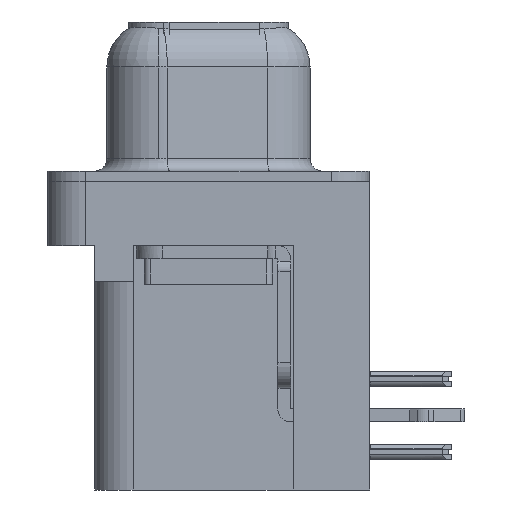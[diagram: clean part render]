
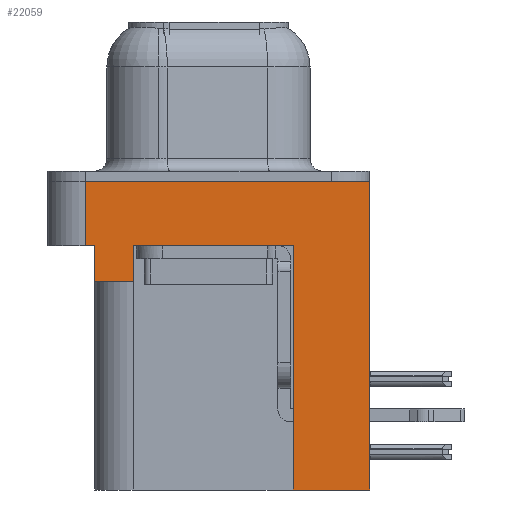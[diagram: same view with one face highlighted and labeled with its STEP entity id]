
A CAD part, left-side view. The second image highlights one B-rep face of the part: STEP entity #22059.
In plain terms, the highlighted planar face has unit normal (-1, 0, 0).
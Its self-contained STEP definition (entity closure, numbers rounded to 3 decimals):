
#230 = DIRECTION ( 'NONE',  ( 0., -1., 0. ) ) ;
#871 = DIRECTION ( 'NONE',  ( -1., 0., 0. ) ) ;
#1240 = DIRECTION ( 'NONE',  ( 0., 0., 1. ) ) ;
#1423 = VECTOR ( 'NONE', #1240, 1000. ) ;
#1454 = LINE ( 'NONE', #35385, #24689 ) ;
#1712 = CARTESIAN_POINT ( 'NONE',  ( -2.91, -3.295, -2.5 ) ) ;
#1952 = VERTEX_POINT ( 'NONE', #25678 ) ;
#1959 = ORIENTED_EDGE ( 'NONE', *, *, #5487, .T. ) ;
#3569 = ORIENTED_EDGE ( 'NONE', *, *, #28888, .F. ) ;
#3679 = LINE ( 'NONE', #10247, #1423 ) ;
#5487 = EDGE_CURVE ( 'NONE', #19455, #36561, #19017, .T. ) ;
#5704 = EDGE_CURVE ( 'NONE', #34224, #36967, #12769, .T. ) ;
#6016 = CARTESIAN_POINT ( 'NONE',  ( -2.91, 2.895, -3.9 ) ) ;
#6312 = EDGE_CURVE ( 'NONE', #34224, #1952, #1454, .T. ) ;
#7328 = EDGE_CURVE ( 'NONE', #1952, #12615, #27888, .T. ) ;
#7333 = EDGE_CURVE ( 'NONE', #30671, #36561, #23378, .T. ) ;
#7464 = DIRECTION ( 'NONE',  ( 0., 0., 1. ) ) ;
#8506 = ORIENTED_EDGE ( 'NONE', *, *, #8767, .F. ) ;
#8767 = EDGE_CURVE ( 'NONE', #19455, #28785, #36981, .T. ) ;
#9227 = ORIENTED_EDGE ( 'NONE', *, *, #5704, .F. ) ;
#9330 = CARTESIAN_POINT ( 'NONE',  ( -2.91, -6.275, 0. ) ) ;
#9486 = VECTOR ( 'NONE', #34793, 1000. ) ;
#9561 = DIRECTION ( 'NONE',  ( 0., 0., 1. ) ) ;
#10042 = VECTOR ( 'NONE', #7464, 1000. ) ;
#10247 = CARTESIAN_POINT ( 'NONE',  ( -2.91, 4.425, -3.9 ) ) ;
#10704 = DIRECTION ( 'NONE',  ( 0., 0., 1. ) ) ;
#10757 = VECTOR ( 'NONE', #230, 1000. ) ;
#11480 = VECTOR ( 'NONE', #15995, 1000. ) ;
#11748 = CARTESIAN_POINT ( 'NONE',  ( -2.91, -6.275, 0. ) ) ;
#12615 = VERTEX_POINT ( 'NONE', #1712 ) ;
#12769 = LINE ( 'NONE', #13774, #26567 ) ;
#12823 = LINE ( 'NONE', #33043, #11480 ) ;
#13774 = CARTESIAN_POINT ( 'NONE',  ( -2.91, 4.425, -3.9 ) ) ;
#14326 = CARTESIAN_POINT ( 'NONE',  ( -2.91, -6.275, -12. ) ) ;
#15126 = ORIENTED_EDGE ( 'NONE', *, *, #29353, .F. ) ;
#15895 = CARTESIAN_POINT ( 'NONE',  ( -2.91, -3.295, -12. ) ) ;
#15995 = DIRECTION ( 'NONE',  ( 0., 0., 1. ) ) ;
#16613 = CARTESIAN_POINT ( 'NONE',  ( -2.91, -6.275, -2.5 ) ) ;
#17686 = VECTOR ( 'NONE', #23473, 1000. ) ;
#18328 = DIRECTION ( 'NONE',  ( 0., 0., 1. ) ) ;
#18672 = ORIENTED_EDGE ( 'NONE', *, *, #7328, .T. ) ;
#18876 = EDGE_LOOP ( 'NONE', ( #28643, #3569, #27681, #15126, #9227, #35859, #18672, #29446, #8506, #1959 ) ) ;
#19017 = LINE ( 'NONE', #16613, #10042 ) ;
#19229 = CARTESIAN_POINT ( 'NONE',  ( -2.91, 4.775, -2.5 ) ) ;
#19455 = VERTEX_POINT ( 'NONE', #14326 ) ;
#20307 = VECTOR ( 'NONE', #10704, 1000. ) ;
#20848 = CARTESIAN_POINT ( 'NONE',  ( -2.91, -6.275, -2.5 ) ) ;
#21636 = FACE_OUTER_BOUND ( 'NONE', #18876, .T. ) ;
#22059 = ADVANCED_FACE ( 'NONE', ( #21636 ), #29882, .T. ) ;
#22552 = CARTESIAN_POINT ( 'NONE',  ( -2.91, -6.275, -2.5 ) ) ;
#23011 = AXIS2_PLACEMENT_3D ( 'NONE', #35419, #871, #9561 ) ;
#23378 = LINE ( 'NONE', #9330, #9486 ) ;
#23473 = DIRECTION ( 'NONE',  ( 0., -1., 0. ) ) ;
#23912 = EDGE_CURVE ( 'NONE', #27477, #36589, #28169, .T. ) ;
#24689 = VECTOR ( 'NONE', #18328, 1000. ) ;
#24942 = DIRECTION ( 'NONE',  ( 0., 1., 0. ) ) ;
#25678 = CARTESIAN_POINT ( 'NONE',  ( -2.91, 2.895, -2.5 ) ) ;
#26457 = CARTESIAN_POINT ( 'NONE',  ( -2.91, -3.295, -12. ) ) ;
#26567 = VECTOR ( 'NONE', #24942, 1000. ) ;
#27477 = VERTEX_POINT ( 'NONE', #35112 ) ;
#27681 = ORIENTED_EDGE ( 'NONE', *, *, #23912, .T. ) ;
#27888 = LINE ( 'NONE', #20848, #17686 ) ;
#28169 = LINE ( 'NONE', #22552, #10757 ) ;
#28643 = ORIENTED_EDGE ( 'NONE', *, *, #7333, .F. ) ;
#28785 = VERTEX_POINT ( 'NONE', #15895 ) ;
#28888 = EDGE_CURVE ( 'NONE', #27477, #30671, #30985, .T. ) ;
#28943 = VECTOR ( 'NONE', #29330, 1000. ) ;
#29330 = DIRECTION ( 'NONE',  ( 0., 1., 0. ) ) ;
#29353 = EDGE_CURVE ( 'NONE', #36967, #36589, #3679, .T. ) ;
#29446 = ORIENTED_EDGE ( 'NONE', *, *, #31472, .F. ) ;
#29882 = PLANE ( 'NONE',  #23011 ) ;
#30671 = VERTEX_POINT ( 'NONE', #34780 ) ;
#30985 = LINE ( 'NONE', #19229, #20307 ) ;
#31472 = EDGE_CURVE ( 'NONE', #28785, #12615, #12823, .T. ) ;
#31695 = CARTESIAN_POINT ( 'NONE',  ( -2.91, 4.425, -2.5 ) ) ;
#33043 = CARTESIAN_POINT ( 'NONE',  ( -2.91, -3.295, -12. ) ) ;
#34040 = CARTESIAN_POINT ( 'NONE',  ( -2.91, 4.425, -3.9 ) ) ;
#34224 = VERTEX_POINT ( 'NONE', #6016 ) ;
#34780 = CARTESIAN_POINT ( 'NONE',  ( -2.91, 4.775, 0. ) ) ;
#34793 = DIRECTION ( 'NONE',  ( 0., -1., 0. ) ) ;
#35112 = CARTESIAN_POINT ( 'NONE',  ( -2.91, 4.775, -2.5 ) ) ;
#35385 = CARTESIAN_POINT ( 'NONE',  ( -2.91, 2.895, -3.9 ) ) ;
#35419 = CARTESIAN_POINT ( 'NONE',  ( -2.91, -6.275, -2.5 ) ) ;
#35859 = ORIENTED_EDGE ( 'NONE', *, *, #6312, .T. ) ;
#36561 = VERTEX_POINT ( 'NONE', #11748 ) ;
#36589 = VERTEX_POINT ( 'NONE', #31695 ) ;
#36967 = VERTEX_POINT ( 'NONE', #34040 ) ;
#36981 = LINE ( 'NONE', #26457, #28943 ) ;
